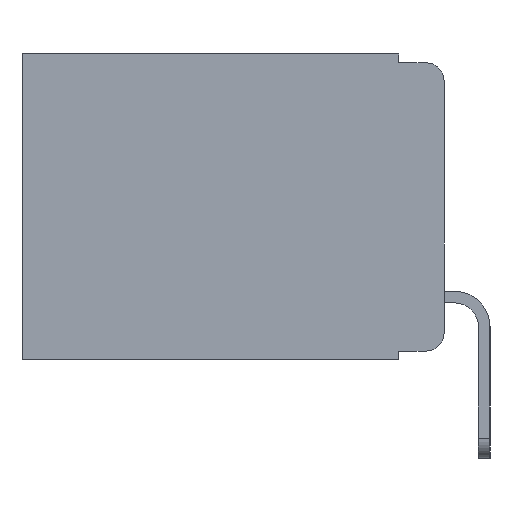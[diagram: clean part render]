
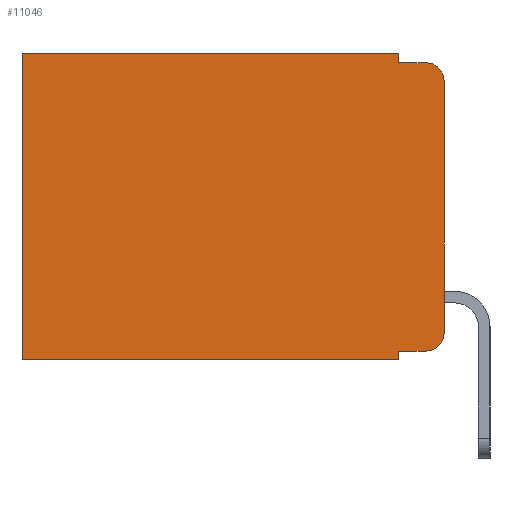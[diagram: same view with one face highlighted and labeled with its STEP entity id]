
A CAD part, left-side view. The second image highlights one B-rep face of the part: STEP entity #11046.
In plain terms, the highlighted planar face has unit normal (-1, 0, 0).
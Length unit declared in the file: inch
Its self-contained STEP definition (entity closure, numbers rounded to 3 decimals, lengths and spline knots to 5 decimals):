
#362 = LINE ( 'NONE', #3772, #10465 ) ;
#1179 = DIRECTION ( 'NONE',  ( 0., 0., -1. ) ) ;
#1308 = ORIENTED_EDGE ( 'NONE', *, *, #19441, .T. ) ;
#1554 = EDGE_CURVE ( 'NONE', #2959, #6203, #3891, .T. ) ;
#2323 = LINE ( 'NONE', #18234, #12348 ) ;
#2781 = VECTOR ( 'NONE', #15477, 39.37008 ) ;
#2918 = ORIENTED_EDGE ( 'NONE', *, *, #10267, .F. ) ;
#2959 = VERTEX_POINT ( 'NONE', #3813 ) ;
#3254 = VERTEX_POINT ( 'NONE', #13403 ) ;
#3266 = VERTEX_POINT ( 'NONE', #13247 ) ;
#3772 = CARTESIAN_POINT ( 'NONE',  ( 0.298, 0.051, -0.333 ) ) ;
#3813 = CARTESIAN_POINT ( 'NONE',  ( 0.298, 0., -0.03 ) ) ;
#3891 = CIRCLE ( 'NONE', #9231, 0.02 ) ;
#3898 = ORIENTED_EDGE ( 'NONE', *, *, #15291, .F. ) ;
#4579 = DIRECTION ( 'NONE',  ( 0., 0., -1. ) ) ;
#4730 = VECTOR ( 'NONE', #4579, 39.37008 ) ;
#4828 = LINE ( 'NONE', #22839, #23713 ) ;
#5505 = LINE ( 'NONE', #9302, #10166 ) ;
#5603 = CARTESIAN_POINT ( 'NONE',  ( 0.298, 0.02, -0.313 ) ) ;
#5666 = CARTESIAN_POINT ( 'NONE',  ( 0.298, 0., 0. ) ) ;
#5857 = DIRECTION ( 'NONE',  ( 0., -1., 0. ) ) ;
#6203 = VERTEX_POINT ( 'NONE', #23623 ) ;
#6298 = VERTEX_POINT ( 'NONE', #15542 ) ;
#7537 = DIRECTION ( 'NONE',  ( -1., 0., 0. ) ) ;
#7662 = DIRECTION ( 'NONE',  ( 0., 0., -1. ) ) ;
#7803 = DIRECTION ( 'NONE',  ( 0., 0., -1. ) ) ;
#8072 = ORIENTED_EDGE ( 'NONE', *, *, #23962, .F. ) ;
#8278 = LINE ( 'NONE', #9780, #2781 ) ;
#8668 = CARTESIAN_POINT ( 'NONE',  ( 0.298, 0., 0. ) ) ;
#8708 = ORIENTED_EDGE ( 'NONE', *, *, #21351, .F. ) ;
#9099 = CARTESIAN_POINT ( 'NONE',  ( 0.298, 0.051, -0.333 ) ) ;
#9231 = AXIS2_PLACEMENT_3D ( 'NONE', #14903, #7537, #22700 ) ;
#9302 = CARTESIAN_POINT ( 'NONE',  ( 0.298, 0.051, 0. ) ) ;
#9425 = LINE ( 'NONE', #8668, #4730 ) ;
#9780 = CARTESIAN_POINT ( 'NONE',  ( 0.298, 0., 0. ) ) ;
#10166 = VECTOR ( 'NONE', #1179, 39.37008 ) ;
#10208 = CARTESIAN_POINT ( 'NONE',  ( 0.298, 0.473, 0. ) ) ;
#10267 = EDGE_CURVE ( 'NONE', #16875, #6298, #14246, .T. ) ;
#10465 = VECTOR ( 'NONE', #5857, 39.37008 ) ;
#10932 = CARTESIAN_POINT ( 'NONE',  ( 0.298, 0.473, -0.343 ) ) ;
#11046 = ADVANCED_FACE ( 'NONE', ( #15101 ), #15371, .F. ) ;
#11390 = AXIS2_PLACEMENT_3D ( 'NONE', #5603, #18949, #7662 ) ;
#12136 = DIRECTION ( 'NONE',  ( 0., 0., -1. ) ) ;
#12348 = VECTOR ( 'NONE', #20070, 39.37008 ) ;
#12774 = LINE ( 'NONE', #10208, #21991 ) ;
#12902 = EDGE_CURVE ( 'NONE', #16875, #20886, #362, .T. ) ;
#13247 = CARTESIAN_POINT ( 'NONE',  ( 0.298, 0.473, 0. ) ) ;
#13403 = CARTESIAN_POINT ( 'NONE',  ( 0.298, 0.051, 0. ) ) ;
#13467 = VERTEX_POINT ( 'NONE', #20725 ) ;
#14246 = LINE ( 'NONE', #23696, #23384 ) ;
#14903 = CARTESIAN_POINT ( 'NONE',  ( 0.298, 0.02, -0.03 ) ) ;
#15101 = FACE_OUTER_BOUND ( 'NONE', #17738, .T. ) ;
#15291 = EDGE_CURVE ( 'NONE', #2959, #13467, #9425, .T. ) ;
#15371 = PLANE ( 'NONE',  #20337 ) ;
#15477 = DIRECTION ( 'NONE',  ( 0., 1., 0. ) ) ;
#15542 = CARTESIAN_POINT ( 'NONE',  ( 0.298, 0.051, -0.343 ) ) ;
#15673 = CIRCLE ( 'NONE', #11390, 0.02 ) ;
#16791 = CARTESIAN_POINT ( 'NONE',  ( 0.298, 0.02, -0.333 ) ) ;
#16875 = VERTEX_POINT ( 'NONE', #9099 ) ;
#17231 = ORIENTED_EDGE ( 'NONE', *, *, #12902, .T. ) ;
#17738 = EDGE_LOOP ( 'NONE', ( #3898, #23727, #8072, #24618, #22343, #1308, #8708, #2918, #17231, #23767 ) ) ;
#17765 = VERTEX_POINT ( 'NONE', #19538 ) ;
#18086 = EDGE_CURVE ( 'NONE', #3254, #17765, #5505, .T. ) ;
#18234 = CARTESIAN_POINT ( 'NONE',  ( 0.298, 0., -0.343 ) ) ;
#18949 = DIRECTION ( 'NONE',  ( -1., 0., 0. ) ) ;
#19078 = DIRECTION ( 'NONE',  ( 1., 0., 0. ) ) ;
#19210 = DIRECTION ( 'NONE',  ( 0., -1., 0. ) ) ;
#19441 = EDGE_CURVE ( 'NONE', #3266, #19574, #12774, .T. ) ;
#19538 = CARTESIAN_POINT ( 'NONE',  ( 0.298, 0.051, -0.01 ) ) ;
#19574 = VERTEX_POINT ( 'NONE', #10932 ) ;
#19758 = EDGE_CURVE ( 'NONE', #20886, #13467, #15673, .T. ) ;
#19811 = EDGE_CURVE ( 'NONE', #3254, #3266, #8278, .T. ) ;
#20070 = DIRECTION ( 'NONE',  ( 0., 1., 0. ) ) ;
#20337 = AXIS2_PLACEMENT_3D ( 'NONE', #5666, #19078, #7803 ) ;
#20725 = CARTESIAN_POINT ( 'NONE',  ( 0.298, 0., -0.313 ) ) ;
#20886 = VERTEX_POINT ( 'NONE', #16791 ) ;
#21351 = EDGE_CURVE ( 'NONE', #6298, #19574, #2323, .T. ) ;
#21881 = DIRECTION ( 'NONE',  ( 0., 0., -1. ) ) ;
#21991 = VECTOR ( 'NONE', #12136, 39.37008 ) ;
#22343 = ORIENTED_EDGE ( 'NONE', *, *, #19811, .T. ) ;
#22700 = DIRECTION ( 'NONE',  ( 0., 0., -1. ) ) ;
#22839 = CARTESIAN_POINT ( 'NONE',  ( 0.298, 0.051, -0.01 ) ) ;
#23384 = VECTOR ( 'NONE', #21881, 39.37008 ) ;
#23623 = CARTESIAN_POINT ( 'NONE',  ( 0.298, 0.02, -0.01 ) ) ;
#23696 = CARTESIAN_POINT ( 'NONE',  ( 0.298, 0.051, 0. ) ) ;
#23713 = VECTOR ( 'NONE', #19210, 39.37008 ) ;
#23727 = ORIENTED_EDGE ( 'NONE', *, *, #1554, .T. ) ;
#23767 = ORIENTED_EDGE ( 'NONE', *, *, #19758, .T. ) ;
#23962 = EDGE_CURVE ( 'NONE', #17765, #6203, #4828, .T. ) ;
#24618 = ORIENTED_EDGE ( 'NONE', *, *, #18086, .F. ) ;
